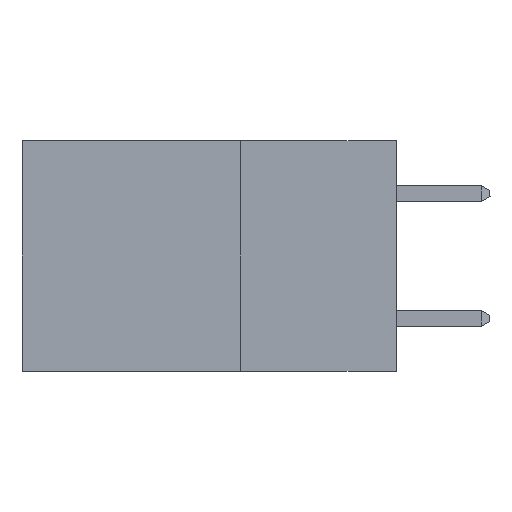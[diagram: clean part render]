
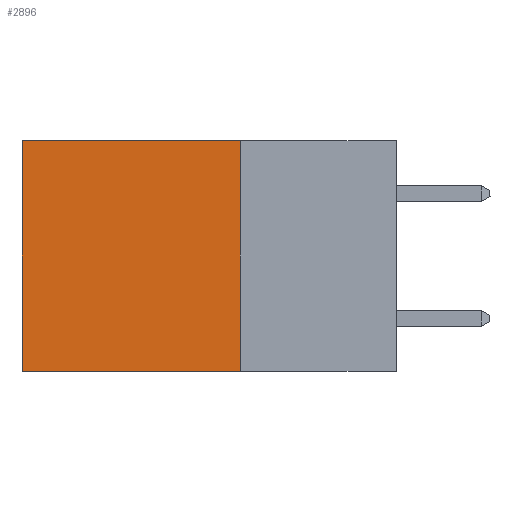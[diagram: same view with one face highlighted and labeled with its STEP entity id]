
A CAD part, left-side view. The second image highlights one B-rep face of the part: STEP entity #2896.
In plain terms, the highlighted planar face has unit normal (-1, 0, 0).
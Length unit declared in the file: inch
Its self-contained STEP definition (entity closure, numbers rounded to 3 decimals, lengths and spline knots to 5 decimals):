
#260 = CARTESIAN_POINT ( 'NONE',  ( 0.298, 0.25, 0. ) ) ;
#616 = DIRECTION ( 'NONE',  ( 0., 0., -1. ) ) ;
#625 = VECTOR ( 'NONE', #16847, 39.37008 ) ;
#1120 = LINE ( 'NONE', #7551, #16278 ) ;
#2896 = ADVANCED_FACE ( 'NONE', ( #18773 ), #18963, .F. ) ;
#3549 = DIRECTION ( 'NONE',  ( 0., 1., 0. ) ) ;
#4339 = CARTESIAN_POINT ( 'NONE',  ( 0.298, 0.25, -0.37 ) ) ;
#5682 = VERTEX_POINT ( 'NONE', #25481 ) ;
#6507 = CARTESIAN_POINT ( 'NONE',  ( 0.298, 0.6, -0.37 ) ) ;
#6702 = LINE ( 'NONE', #16932, #625 ) ;
#7449 = EDGE_CURVE ( 'NONE', #5682, #24041, #6702, .T. ) ;
#7551 = CARTESIAN_POINT ( 'NONE',  ( 0.298, 0.25, -0.37 ) ) ;
#7724 = VERTEX_POINT ( 'NONE', #6507 ) ;
#9311 = CARTESIAN_POINT ( 'NONE',  ( 0.298, 0.25, 0. ) ) ;
#9426 = AXIS2_PLACEMENT_3D ( 'NONE', #9311, #16676, #16753 ) ;
#10551 = EDGE_CURVE ( 'NONE', #22092, #7724, #1120, .T. ) ;
#11701 = LINE ( 'NONE', #17090, #16630 ) ;
#12558 = DIRECTION ( 'NONE',  ( 0., 0., -1. ) ) ;
#12575 = ORIENTED_EDGE ( 'NONE', *, *, #23077, .F. ) ;
#14585 = EDGE_CURVE ( 'NONE', #24041, #7724, #11701, .T. ) ;
#15670 = ORIENTED_EDGE ( 'NONE', *, *, #7449, .T. ) ;
#16008 = ORIENTED_EDGE ( 'NONE', *, *, #14585, .T. ) ;
#16278 = VECTOR ( 'NONE', #3549, 39.37008 ) ;
#16630 = VECTOR ( 'NONE', #616, 39.37008 ) ;
#16676 = DIRECTION ( 'NONE',  ( 1., 0., 0. ) ) ;
#16753 = DIRECTION ( 'NONE',  ( 0., 0., -1. ) ) ;
#16847 = DIRECTION ( 'NONE',  ( 0., 1., 0. ) ) ;
#16932 = CARTESIAN_POINT ( 'NONE',  ( 0.298, 0.25, 0. ) ) ;
#17090 = CARTESIAN_POINT ( 'NONE',  ( 0.298, 0.6, 0. ) ) ;
#17719 = ORIENTED_EDGE ( 'NONE', *, *, #10551, .F. ) ;
#18773 = FACE_OUTER_BOUND ( 'NONE', #23956, .T. ) ;
#18963 = PLANE ( 'NONE',  #9426 ) ;
#20560 = VECTOR ( 'NONE', #12558, 39.37008 ) ;
#22092 = VERTEX_POINT ( 'NONE', #4339 ) ;
#23077 = EDGE_CURVE ( 'NONE', #5682, #22092, #23862, .T. ) ;
#23136 = CARTESIAN_POINT ( 'NONE',  ( 0.298, 0.6, 0. ) ) ;
#23862 = LINE ( 'NONE', #260, #20560 ) ;
#23956 = EDGE_LOOP ( 'NONE', ( #16008, #17719, #12575, #15670 ) ) ;
#24041 = VERTEX_POINT ( 'NONE', #23136 ) ;
#25481 = CARTESIAN_POINT ( 'NONE',  ( 0.298, 0.25, 0. ) ) ;
